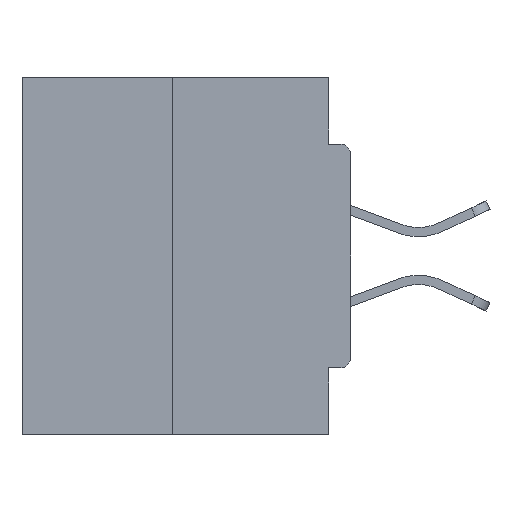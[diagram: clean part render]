
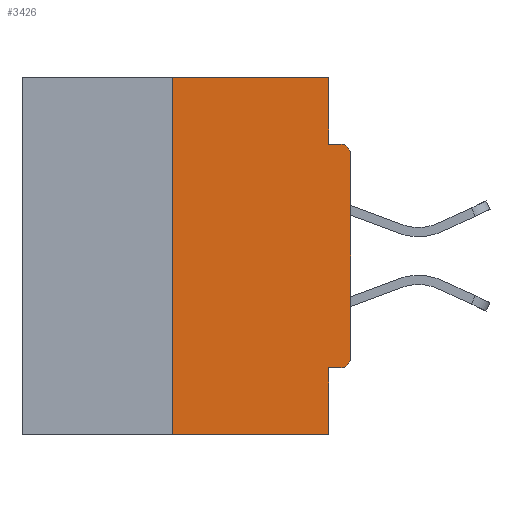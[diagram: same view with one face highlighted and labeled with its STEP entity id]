
A CAD part, left-side view. The second image highlights one B-rep face of the part: STEP entity #3426.
In plain terms, the highlighted planar face has unit normal (-1, 0, 0).
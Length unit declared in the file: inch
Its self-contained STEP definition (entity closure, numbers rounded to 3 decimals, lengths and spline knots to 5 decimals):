
#273 = LINE ( 'NONE', #9090, #2540 ) ;
#886 = DIRECTION ( 'NONE',  ( 0., 0., -1. ) ) ;
#1004 = ORIENTED_EDGE ( 'NONE', *, *, #18265, .T. ) ;
#1979 = VECTOR ( 'NONE', #26774, 39.37008 ) ;
#2522 = LINE ( 'NONE', #26141, #8910 ) ;
#2540 = VECTOR ( 'NONE', #38786, 39.37008 ) ;
#3398 = ORIENTED_EDGE ( 'NONE', *, *, #15347, .F. ) ;
#3425 = DIRECTION ( 'NONE',  ( 0., 0., 1. ) ) ;
#3426 = ADVANCED_FACE ( 'NONE', ( #30685 ), #17282, .F. ) ;
#4815 = LINE ( 'NONE', #5895, #33743 ) ;
#5491 = VERTEX_POINT ( 'NONE', #7057 ) ;
#5795 = ORIENTED_EDGE ( 'NONE', *, *, #47325, .F. ) ;
#5895 = CARTESIAN_POINT ( 'NONE',  ( 0., 0.031, 0. ) ) ;
#6141 = VERTEX_POINT ( 'NONE', #42368 ) ;
#6568 = CARTESIAN_POINT ( 'NONE',  ( 0., 0.25, -0.5 ) ) ;
#6632 = VERTEX_POINT ( 'NONE', #19859 ) ;
#6803 = CARTESIAN_POINT ( 'NONE',  ( 0., 0.031, 0. ) ) ;
#6964 = EDGE_CURVE ( 'NONE', #26635, #6632, #42521, .T. ) ;
#7057 = CARTESIAN_POINT ( 'NONE',  ( 0., 0.031, -0.4065 ) ) ;
#7975 = VERTEX_POINT ( 'NONE', #6568 ) ;
#8329 = LINE ( 'NONE', #41798, #1979 ) ;
#8910 = VECTOR ( 'NONE', #15615, 39.37008 ) ;
#9090 = CARTESIAN_POINT ( 'NONE',  ( 0., 0.46, 0. ) ) ;
#9563 = VECTOR ( 'NONE', #886, 39.37008 ) ;
#9655 = DIRECTION ( 'NONE',  ( 0., 0., -1. ) ) ;
#10155 = CARTESIAN_POINT ( 'NONE',  ( 0., 0.015, -0.0935 ) ) ;
#10474 = VERTEX_POINT ( 'NONE', #34616 ) ;
#10699 = VERTEX_POINT ( 'NONE', #10155 ) ;
#11340 = CARTESIAN_POINT ( 'NONE',  ( 0., 0.015, -0.1085 ) ) ;
#12769 = EDGE_LOOP ( 'NONE', ( #5795, #39572, #1004, #15724, #3398, #17419, #40370, #36279, #30255, #35334 ) ) ;
#14367 = EDGE_CURVE ( 'NONE', #43453, #26635, #47182, .T. ) ;
#15338 = AXIS2_PLACEMENT_3D ( 'NONE', #42738, #45968, #31226 ) ;
#15347 = EDGE_CURVE ( 'NONE', #43453, #5491, #8329, .T. ) ;
#15533 = EDGE_CURVE ( 'NONE', #17240, #6141, #4815, .T. ) ;
#15615 = DIRECTION ( 'NONE',  ( 0., -1., 0. ) ) ;
#15724 = ORIENTED_EDGE ( 'NONE', *, *, #31966, .F. ) ;
#15878 = CARTESIAN_POINT ( 'NONE',  ( 0., 0.031, -0.5 ) ) ;
#17240 = VERTEX_POINT ( 'NONE', #6803 ) ;
#17282 = PLANE ( 'NONE',  #32300 ) ;
#17419 = ORIENTED_EDGE ( 'NONE', *, *, #14367, .T. ) ;
#18265 = EDGE_CURVE ( 'NONE', #7975, #27747, #39340, .T. ) ;
#19859 = CARTESIAN_POINT ( 'NONE',  ( 0., 0., -0.1085 ) ) ;
#20978 = EDGE_CURVE ( 'NONE', #6141, #10699, #2522, .T. ) ;
#22321 = DIRECTION ( 'NONE',  ( -1., 0., 0. ) ) ;
#24124 = DIRECTION ( 'NONE',  ( 0., -1., 0. ) ) ;
#24557 = DIRECTION ( 'NONE',  ( 1., 0., 0. ) ) ;
#26029 = DIRECTION ( 'NONE',  ( 0., 0., -1. ) ) ;
#26141 = CARTESIAN_POINT ( 'NONE',  ( 0., 0., -0.0935 ) ) ;
#26283 = CARTESIAN_POINT ( 'NONE',  ( 0., 0., -0.3915 ) ) ;
#26635 = VERTEX_POINT ( 'NONE', #26283 ) ;
#26774 = DIRECTION ( 'NONE',  ( 0., 1., 0. ) ) ;
#27309 = LINE ( 'NONE', #38541, #45809 ) ;
#27442 = LINE ( 'NONE', #37856, #9563 ) ;
#27565 = DIRECTION ( 'NONE',  ( 0., 0., 1. ) ) ;
#27607 = EDGE_CURVE ( 'NONE', #7975, #10474, #27309, .T. ) ;
#27747 = VERTEX_POINT ( 'NONE', #15878 ) ;
#30255 = ORIENTED_EDGE ( 'NONE', *, *, #20978, .F. ) ;
#30685 = FACE_OUTER_BOUND ( 'NONE', #12769, .T. ) ;
#31226 = DIRECTION ( 'NONE',  ( 0., 0., -1. ) ) ;
#31516 = VECTOR ( 'NONE', #3425, 39.37008 ) ;
#31966 = EDGE_CURVE ( 'NONE', #5491, #27747, #27442, .T. ) ;
#32300 = AXIS2_PLACEMENT_3D ( 'NONE', #46683, #24557, #43126 ) ;
#32519 = CARTESIAN_POINT ( 'NONE',  ( 0., 0.015, -0.4065 ) ) ;
#33743 = VECTOR ( 'NONE', #9655, 39.37008 ) ;
#34616 = CARTESIAN_POINT ( 'NONE',  ( 0., 0.25, 0. ) ) ;
#35334 = ORIENTED_EDGE ( 'NONE', *, *, #15533, .F. ) ;
#36279 = ORIENTED_EDGE ( 'NONE', *, *, #45216, .T. ) ;
#37856 = CARTESIAN_POINT ( 'NONE',  ( 0., 0.031, -0.5 ) ) ;
#38167 = VECTOR ( 'NONE', #24124, 39.37008 ) ;
#38541 = CARTESIAN_POINT ( 'NONE',  ( 0., 0.25, 0. ) ) ;
#38777 = CARTESIAN_POINT ( 'NONE',  ( 0., 0.46, -0.5 ) ) ;
#38786 = DIRECTION ( 'NONE',  ( 0., -1., 0. ) ) ;
#39340 = LINE ( 'NONE', #38777, #38167 ) ;
#39572 = ORIENTED_EDGE ( 'NONE', *, *, #27607, .F. ) ;
#40370 = ORIENTED_EDGE ( 'NONE', *, *, #6964, .T. ) ;
#40954 = CIRCLE ( 'NONE', #42128, 0.015 ) ;
#41798 = CARTESIAN_POINT ( 'NONE',  ( 0., 0., -0.4065 ) ) ;
#42128 = AXIS2_PLACEMENT_3D ( 'NONE', #11340, #22321, #26029 ) ;
#42368 = CARTESIAN_POINT ( 'NONE',  ( 0., 0.031, -0.0935 ) ) ;
#42521 = LINE ( 'NONE', #44167, #31516 ) ;
#42738 = CARTESIAN_POINT ( 'NONE',  ( 0., 0.015, -0.3915 ) ) ;
#43126 = DIRECTION ( 'NONE',  ( 0., 0., -1. ) ) ;
#43453 = VERTEX_POINT ( 'NONE', #32519 ) ;
#44167 = CARTESIAN_POINT ( 'NONE',  ( 0., 0., 0. ) ) ;
#45216 = EDGE_CURVE ( 'NONE', #6632, #10699, #40954, .T. ) ;
#45809 = VECTOR ( 'NONE', #27565, 39.37008 ) ;
#45968 = DIRECTION ( 'NONE',  ( -1., 0., 0. ) ) ;
#46683 = CARTESIAN_POINT ( 'NONE',  ( 0., 0.46, 0. ) ) ;
#47182 = CIRCLE ( 'NONE', #15338, 0.015 ) ;
#47325 = EDGE_CURVE ( 'NONE', #10474, #17240, #273, .T. ) ;
